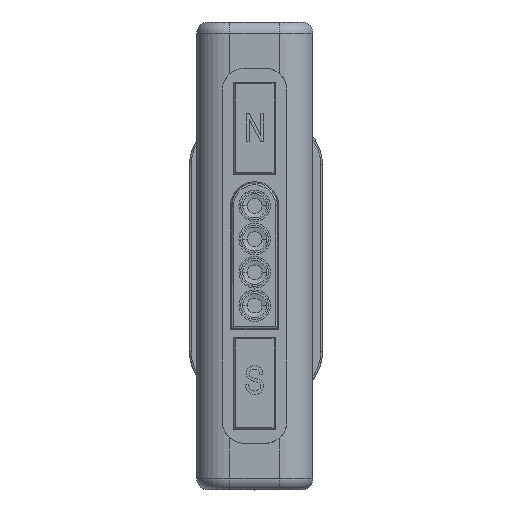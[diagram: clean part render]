
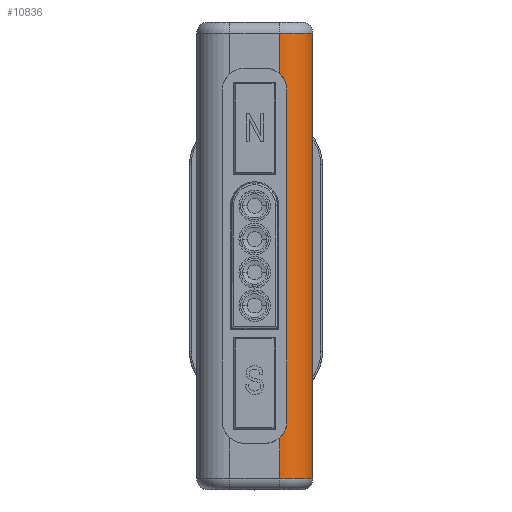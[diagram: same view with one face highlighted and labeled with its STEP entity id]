
A CAD part, top view. The second image highlights one B-rep face of the part: STEP entity #10836.
In plain terms, the highlighted cylindrical face has radius 1.8 mm (diameter 3.6 mm), a partial arc.
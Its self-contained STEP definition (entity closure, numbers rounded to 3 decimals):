
#150 = CARTESIAN_POINT ( 'NONE',  ( 1.345, 12.65, 6.8 ) ) ;
#423 = VECTOR ( 'NONE', #11213, 1000. ) ;
#489 = LINE ( 'NONE', #10503, #1454 ) ;
#586 = ORIENTED_EDGE ( 'NONE', *, *, #5318, .T. ) ;
#680 = LINE ( 'NONE', #11410, #423 ) ;
#1003 = EDGE_CURVE ( 'NONE', #10718, #10595, #10258, .T. ) ;
#1034 = ORIENTED_EDGE ( 'NONE', *, *, #4703, .T. ) ;
#1434 = DIRECTION ( 'NONE',  ( 0., -1., 0. ) ) ;
#1454 = VECTOR ( 'NONE', #8401, 1000. ) ;
#1836 = CIRCLE ( 'NONE', #7656, 1.8 ) ;
#2095 = CARTESIAN_POINT ( 'NONE',  ( 1.345, 12.05, 5. ) ) ;
#2108 = LINE ( 'NONE', #150, #6020 ) ;
#2170 = VERTEX_POINT ( 'NONE', #11799 ) ;
#2225 = VERTEX_POINT ( 'NONE', #5160 ) ;
#2573 = CIRCLE ( 'NONE', #12410, 1.8 ) ;
#2594 = ORIENTED_EDGE ( 'NONE', *, *, #11767, .T. ) ;
#2619 = CYLINDRICAL_SURFACE ( 'NONE', #4666, 1.8 ) ;
#2674 = FACE_OUTER_BOUND ( 'NONE', #12081, .T. ) ;
#2763 = ORIENTED_EDGE ( 'NONE', *, *, #4681, .F. ) ;
#3052 = DIRECTION ( 'NONE',  ( 0., -1., 0. ) ) ;
#3107 = CARTESIAN_POINT ( 'NONE',  ( 1.345, -12.05, 5. ) ) ;
#3440 = CARTESIAN_POINT ( 'NONE',  ( 1.345, -9.849, 6.8 ) ) ;
#3899 = DIRECTION ( 'NONE',  ( 0., 0., -1. ) ) ;
#4274 = CARTESIAN_POINT ( 'NONE',  ( 1.345, 12.65, 6.8 ) ) ;
#4337 = EDGE_CURVE ( 'NONE', #2170, #10718, #1836, .T. ) ;
#4501 = CARTESIAN_POINT ( 'NONE',  ( 1.345, -12.05, 6.8 ) ) ;
#4666 = AXIS2_PLACEMENT_3D ( 'NONE', #11322, #11199, #10431 ) ;
#4681 = EDGE_CURVE ( 'NONE', #2170, #2225, #680, .T. ) ;
#4703 = EDGE_CURVE ( 'NONE', #9401, #7657, #489, .T. ) ;
#5061 = DIRECTION ( 'NONE',  ( 0., 1., 0. ) ) ;
#5160 = CARTESIAN_POINT ( 'NONE',  ( 3.145, -12.05, 5. ) ) ;
#5318 = EDGE_CURVE ( 'NONE', #10595, #9401, #2108, .T. ) ;
#6020 = VECTOR ( 'NONE', #3052, 1000. ) ;
#7047 = VECTOR ( 'NONE', #1434, 1000. ) ;
#7656 = AXIS2_PLACEMENT_3D ( 'NONE', #2095, #9840, #10709 ) ;
#7657 = VERTEX_POINT ( 'NONE', #4501 ) ;
#8401 = DIRECTION ( 'NONE',  ( 0., -1., 0. ) ) ;
#9373 = CARTESIAN_POINT ( 'NONE',  ( 1.345, 12.05, 6.8 ) ) ;
#9401 = VERTEX_POINT ( 'NONE', #3440 ) ;
#9840 = DIRECTION ( 'NONE',  ( 0., -1., 0. ) ) ;
#10258 = LINE ( 'NONE', #4274, #7047 ) ;
#10431 = DIRECTION ( 'NONE',  ( 0., 0., -1. ) ) ;
#10503 = CARTESIAN_POINT ( 'NONE',  ( 1.345, 12.65, 6.8 ) ) ;
#10595 = VERTEX_POINT ( 'NONE', #12563 ) ;
#10661 = ORIENTED_EDGE ( 'NONE', *, *, #4337, .T. ) ;
#10709 = DIRECTION ( 'NONE',  ( 0., 0., -1. ) ) ;
#10718 = VERTEX_POINT ( 'NONE', #9373 ) ;
#10836 = ADVANCED_FACE ( 'NONE', ( #2674 ), #2619, .T. ) ;
#11199 = DIRECTION ( 'NONE',  ( 0., -1., 0. ) ) ;
#11213 = DIRECTION ( 'NONE',  ( 0., -1., 0. ) ) ;
#11322 = CARTESIAN_POINT ( 'NONE',  ( 1.345, 12.65, 5. ) ) ;
#11410 = CARTESIAN_POINT ( 'NONE',  ( 3.145, 12.65, 5. ) ) ;
#11767 = EDGE_CURVE ( 'NONE', #7657, #2225, #2573, .T. ) ;
#11799 = CARTESIAN_POINT ( 'NONE',  ( 3.145, 12.05, 5. ) ) ;
#11902 = ORIENTED_EDGE ( 'NONE', *, *, #1003, .T. ) ;
#12081 = EDGE_LOOP ( 'NONE', ( #1034, #2594, #2763, #10661, #11902, #586 ) ) ;
#12410 = AXIS2_PLACEMENT_3D ( 'NONE', #3107, #5061, #3899 ) ;
#12563 = CARTESIAN_POINT ( 'NONE',  ( 1.345, 9.849, 6.8 ) ) ;
